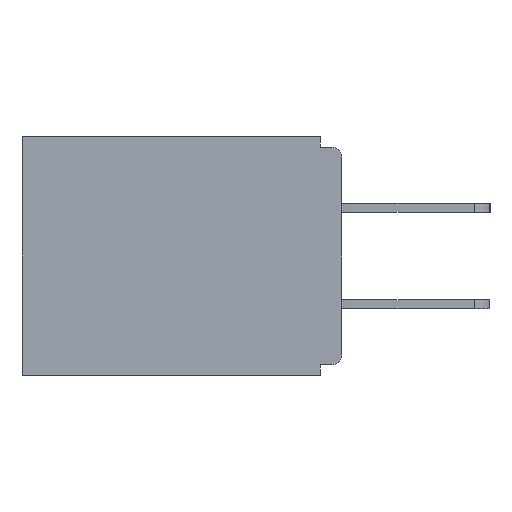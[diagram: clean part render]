
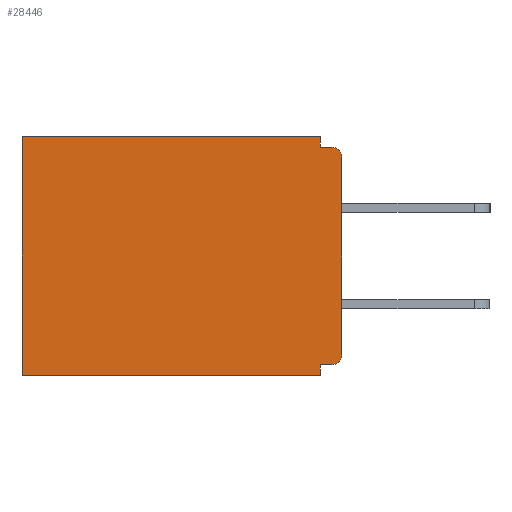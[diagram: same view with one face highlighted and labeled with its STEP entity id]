
A CAD part, left-side view. The second image highlights one B-rep face of the part: STEP entity #28446.
In plain terms, the highlighted planar face has unit normal (-1, 0, 0).
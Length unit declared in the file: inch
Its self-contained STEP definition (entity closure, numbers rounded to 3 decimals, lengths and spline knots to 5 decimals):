
#242 = EDGE_CURVE ( 'NONE', #26626, #2521, #7526, .T. ) ;
#436 = CARTESIAN_POINT ( 'NONE',  ( 0.298, 0., -0.328 ) ) ;
#911 = VECTOR ( 'NONE', #20278, 39.37008 ) ;
#1225 = FACE_OUTER_BOUND ( 'NONE', #22134, .T. ) ;
#1458 = CARTESIAN_POINT ( 'NONE',  ( 0.298, 0.46, 0. ) ) ;
#2099 = DIRECTION ( 'NONE',  ( 0., -1., 0. ) ) ;
#2521 = VERTEX_POINT ( 'NONE', #26520 ) ;
#2571 = EDGE_CURVE ( 'NONE', #23984, #26626, #19581, .T. ) ;
#3898 = CARTESIAN_POINT ( 'NONE',  ( 0.298, 0.015, -0.328 ) ) ;
#4169 = AXIS2_PLACEMENT_3D ( 'NONE', #17073, #17774, #8771 ) ;
#4265 = DIRECTION ( 'NONE',  ( 0., 1., 0. ) ) ;
#5081 = CARTESIAN_POINT ( 'NONE',  ( 0.298, 0.015, -0.03 ) ) ;
#5589 = CARTESIAN_POINT ( 'NONE',  ( 0.298, 0.031, -0.015 ) ) ;
#5828 = LINE ( 'NONE', #19739, #19360 ) ;
#5934 = VECTOR ( 'NONE', #15352, 39.37008 ) ;
#6227 = ORIENTED_EDGE ( 'NONE', *, *, #18445, .F. ) ;
#6479 = CARTESIAN_POINT ( 'NONE',  ( 0.298, 0.031, -0.343 ) ) ;
#6503 = CARTESIAN_POINT ( 'NONE',  ( 0.298, 0.031, 0. ) ) ;
#6969 = VECTOR ( 'NONE', #13398, 39.37008 ) ;
#7103 = DIRECTION ( 'NONE',  ( 0., 0., -1. ) ) ;
#7486 = ORIENTED_EDGE ( 'NONE', *, *, #27066, .T. ) ;
#7526 = LINE ( 'NONE', #21337, #22156 ) ;
#7707 = DIRECTION ( 'NONE',  ( 0., 0., -1. ) ) ;
#7952 = CARTESIAN_POINT ( 'NONE',  ( 0.298, 0.015, -0.015 ) ) ;
#8373 = VERTEX_POINT ( 'NONE', #7952 ) ;
#8460 = DIRECTION ( 'NONE',  ( 0., 1., 0. ) ) ;
#8476 = CARTESIAN_POINT ( 'NONE',  ( 0.298, 0., -0.015 ) ) ;
#8771 = DIRECTION ( 'NONE',  ( 0., 0., -1. ) ) ;
#8812 = CIRCLE ( 'NONE', #27412, 0.015 ) ;
#9165 = EDGE_CURVE ( 'NONE', #19536, #8373, #17115, .T. ) ;
#9572 = VERTEX_POINT ( 'NONE', #3898 ) ;
#9866 = DIRECTION ( 'NONE',  ( 0., 0., -1. ) ) ;
#10064 = ORIENTED_EDGE ( 'NONE', *, *, #13933, .F. ) ;
#10854 = DIRECTION ( 'NONE',  ( 0., 0., -1. ) ) ;
#10866 = VERTEX_POINT ( 'NONE', #6479 ) ;
#11236 = VECTOR ( 'NONE', #4265, 39.37008 ) ;
#11345 = CARTESIAN_POINT ( 'NONE',  ( 0.298, 0., 0. ) ) ;
#11436 = ORIENTED_EDGE ( 'NONE', *, *, #9165, .F. ) ;
#11664 = EDGE_CURVE ( 'NONE', #13509, #8373, #28465, .T. ) ;
#12072 = DIRECTION ( 'NONE',  ( -1., 0., 0. ) ) ;
#12214 = ORIENTED_EDGE ( 'NONE', *, *, #242, .T. ) ;
#12560 = ORIENTED_EDGE ( 'NONE', *, *, #22699, .F. ) ;
#12867 = LINE ( 'NONE', #436, #6969 ) ;
#13069 = CARTESIAN_POINT ( 'NONE',  ( 0.298, 0.031, -0.343 ) ) ;
#13302 = PLANE ( 'NONE',  #4169 ) ;
#13395 = CARTESIAN_POINT ( 'NONE',  ( 0.298, 0.031, -0.328 ) ) ;
#13398 = DIRECTION ( 'NONE',  ( 0., 1., 0. ) ) ;
#13509 = VERTEX_POINT ( 'NONE', #18532 ) ;
#13933 = EDGE_CURVE ( 'NONE', #23984, #19536, #27696, .T. ) ;
#15221 = VERTEX_POINT ( 'NONE', #13395 ) ;
#15299 = CARTESIAN_POINT ( 'NONE',  ( 0.298, 0., -0.313 ) ) ;
#15352 = DIRECTION ( 'NONE',  ( 0., 0., -1. ) ) ;
#15745 = LINE ( 'NONE', #11345, #911 ) ;
#16176 = ORIENTED_EDGE ( 'NONE', *, *, #26265, .F. ) ;
#16525 = VERTEX_POINT ( 'NONE', #15299 ) ;
#17073 = CARTESIAN_POINT ( 'NONE',  ( 0.298, 0., 0. ) ) ;
#17115 = LINE ( 'NONE', #8476, #27607 ) ;
#17774 = DIRECTION ( 'NONE',  ( 1., 0., 0. ) ) ;
#18445 = EDGE_CURVE ( 'NONE', #9572, #15221, #12867, .T. ) ;
#18532 = CARTESIAN_POINT ( 'NONE',  ( 0.298, 0., -0.03 ) ) ;
#19360 = VECTOR ( 'NONE', #8460, 39.37008 ) ;
#19536 = VERTEX_POINT ( 'NONE', #5589 ) ;
#19581 = LINE ( 'NONE', #22042, #11236 ) ;
#19739 = CARTESIAN_POINT ( 'NONE',  ( 0.298, 0., -0.343 ) ) ;
#20278 = DIRECTION ( 'NONE',  ( 0., 0., -1. ) ) ;
#20409 = EDGE_CURVE ( 'NONE', #10866, #2521, #5828, .T. ) ;
#20427 = DIRECTION ( 'NONE',  ( -1., 0., 0. ) ) ;
#20567 = AXIS2_PLACEMENT_3D ( 'NONE', #5081, #20427, #7103 ) ;
#21212 = CARTESIAN_POINT ( 'NONE',  ( 0.298, 0.015, -0.313 ) ) ;
#21337 = CARTESIAN_POINT ( 'NONE',  ( 0.298, 0.46, 0. ) ) ;
#21574 = LINE ( 'NONE', #13069, #5934 ) ;
#22042 = CARTESIAN_POINT ( 'NONE',  ( 0.298, 0., 0. ) ) ;
#22134 = EDGE_LOOP ( 'NONE', ( #24850, #11436, #10064, #25895, #12214, #26675, #12560, #6227, #7486, #16176 ) ) ;
#22156 = VECTOR ( 'NONE', #9866, 39.37008 ) ;
#22699 = EDGE_CURVE ( 'NONE', #15221, #10866, #21574, .T. ) ;
#23984 = VERTEX_POINT ( 'NONE', #6503 ) ;
#24193 = CARTESIAN_POINT ( 'NONE',  ( 0.298, 0.031, -0.343 ) ) ;
#24850 = ORIENTED_EDGE ( 'NONE', *, *, #11664, .T. ) ;
#25895 = ORIENTED_EDGE ( 'NONE', *, *, #2571, .T. ) ;
#26265 = EDGE_CURVE ( 'NONE', #13509, #16525, #15745, .T. ) ;
#26520 = CARTESIAN_POINT ( 'NONE',  ( 0.298, 0.46, -0.343 ) ) ;
#26626 = VERTEX_POINT ( 'NONE', #1458 ) ;
#26675 = ORIENTED_EDGE ( 'NONE', *, *, #20409, .F. ) ;
#27066 = EDGE_CURVE ( 'NONE', #9572, #16525, #8812, .T. ) ;
#27412 = AXIS2_PLACEMENT_3D ( 'NONE', #21212, #12072, #7707 ) ;
#27607 = VECTOR ( 'NONE', #2099, 39.37008 ) ;
#27696 = LINE ( 'NONE', #24193, #28060 ) ;
#28060 = VECTOR ( 'NONE', #10854, 39.37008 ) ;
#28446 = ADVANCED_FACE ( 'NONE', ( #1225 ), #13302, .F. ) ;
#28465 = CIRCLE ( 'NONE', #20567, 0.015 ) ;
